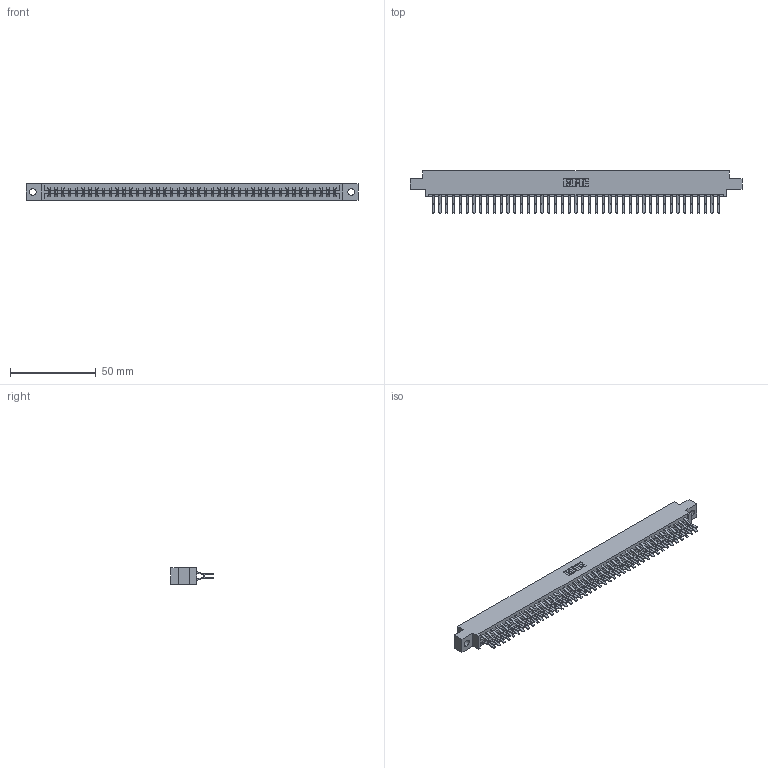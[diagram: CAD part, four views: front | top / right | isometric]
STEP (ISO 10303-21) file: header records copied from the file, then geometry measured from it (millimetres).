
FILE_DESCRIPTION (( 'STEP AP203' ), '1' );
FILE_NAME ('337-086-560-804.STEP', '2018-08-13T02:44:03', ( '' ), ( '' ), 'SwSTEP 2.0', 'SolidWorks 2016', '' );
FILE_SCHEMA (( 'CONFIG_CONTROL_DESIGN' ));
Length unit declared in the file: inch
Products named in the file (3): 337 Part_0.170 Offset - 0.156 Dia-TH; 345-292-001_560 Tail; 337-086-560-804
Assembly tree (87 placements, depth 2):
  337-086-560-804
    337 Part_0.170 Offset - 0.156 Dia-TH
    345-292-001_560 Tail  x86
Bounding box: 193.4 x 24.78 x 9.4 mm (x, y, z)
Volume: 20753.2 mm3; surface area: 25008 mm2
Topology: 87 solids, 87 shells, 4934 faces, 14685 edges, 9674 vertices
Faces by surface type: plane 3342, cylinder 1592
Entity records: 33433 total; most frequent: CARTESIAN_POINT 5634, ORIENTED_EDGE 5570, DIRECTION 4793, EDGE_CURVE 2785, LINE 2653, VECTOR 2653, VERTEX_POINT 1854, AXIS2_PLACEMENT_3D 1070
